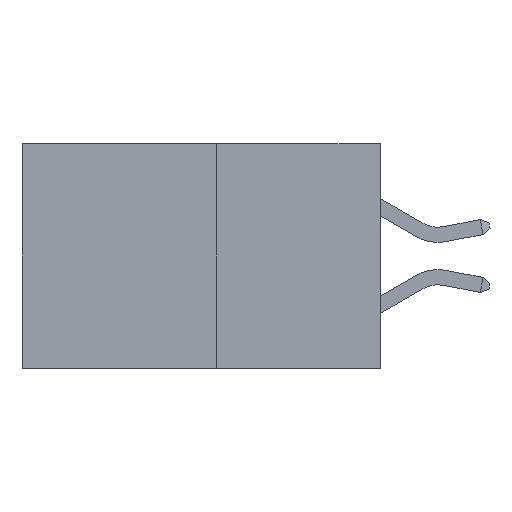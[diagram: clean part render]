
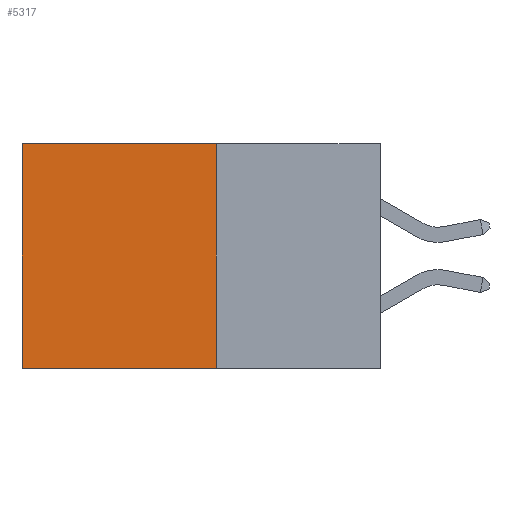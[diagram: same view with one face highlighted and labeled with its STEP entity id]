
A CAD part, left-side view. The second image highlights one B-rep face of the part: STEP entity #5317.
In plain terms, the highlighted planar face has unit normal (-1, 0, 0).
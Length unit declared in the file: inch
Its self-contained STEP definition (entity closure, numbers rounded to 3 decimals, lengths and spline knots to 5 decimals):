
#387 = DIRECTION ( 'NONE',  ( 0., 1., 0. ) ) ;
#841 = VECTOR ( 'NONE', #8076, 39.37008 ) ;
#886 = ORIENTED_EDGE ( 'NONE', *, *, #4565, .F. ) ;
#988 = AXIS2_PLACEMENT_3D ( 'NONE', #6729, #3667, #8965 ) ;
#1126 = VERTEX_POINT ( 'NONE', #8016 ) ;
#1153 = ORIENTED_EDGE ( 'NONE', *, *, #5943, .F. ) ;
#1343 = CARTESIAN_POINT ( 'NONE',  ( 0.277, 0.27, -0.37 ) ) ;
#1361 = ORIENTED_EDGE ( 'NONE', *, *, #4518, .T. ) ;
#2018 = CARTESIAN_POINT ( 'NONE',  ( 0.277, 0.27, -0.37 ) ) ;
#2144 = DIRECTION ( 'NONE',  ( 0., 0., -1. ) ) ;
#2391 = ORIENTED_EDGE ( 'NONE', *, *, #8601, .T. ) ;
#2939 = CARTESIAN_POINT ( 'NONE',  ( 0.277, 0.27, 0. ) ) ;
#3139 = VECTOR ( 'NONE', #387, 39.37008 ) ;
#3479 = CARTESIAN_POINT ( 'NONE',  ( 0.277, 0.59, 0. ) ) ;
#3667 = DIRECTION ( 'NONE',  ( 1., 0., 0. ) ) ;
#3730 = VECTOR ( 'NONE', #9463, 39.37008 ) ;
#3890 = VERTEX_POINT ( 'NONE', #3479 ) ;
#4222 = CARTESIAN_POINT ( 'NONE',  ( 0.277, 0.27, 0. ) ) ;
#4518 = EDGE_CURVE ( 'NONE', #4718, #3890, #5203, .T. ) ;
#4565 = EDGE_CURVE ( 'NONE', #9541, #1126, #6951, .T. ) ;
#4718 = VERTEX_POINT ( 'NONE', #2939 ) ;
#4746 = CARTESIAN_POINT ( 'NONE',  ( 0.277, 0.27, -0.37 ) ) ;
#5203 = LINE ( 'NONE', #4222, #3139 ) ;
#5317 = ADVANCED_FACE ( 'NONE', ( #6820 ), #8253, .F. ) ;
#5498 = LINE ( 'NONE', #1343, #9190 ) ;
#5943 = EDGE_CURVE ( 'NONE', #4718, #9541, #5498, .T. ) ;
#6531 = CARTESIAN_POINT ( 'NONE',  ( 0.277, 0.59, -0.37 ) ) ;
#6729 = CARTESIAN_POINT ( 'NONE',  ( 0.277, 0.27, -0.37 ) ) ;
#6820 = FACE_OUTER_BOUND ( 'NONE', #9131, .T. ) ;
#6951 = LINE ( 'NONE', #2018, #841 ) ;
#7812 = LINE ( 'NONE', #6531, #3730 ) ;
#8016 = CARTESIAN_POINT ( 'NONE',  ( 0.277, 0.59, -0.37 ) ) ;
#8076 = DIRECTION ( 'NONE',  ( 0., 1., 0. ) ) ;
#8253 = PLANE ( 'NONE',  #988 ) ;
#8601 = EDGE_CURVE ( 'NONE', #3890, #1126, #7812, .T. ) ;
#8965 = DIRECTION ( 'NONE',  ( 0., 0., -1. ) ) ;
#9131 = EDGE_LOOP ( 'NONE', ( #2391, #886, #1153, #1361 ) ) ;
#9190 = VECTOR ( 'NONE', #2144, 39.37008 ) ;
#9463 = DIRECTION ( 'NONE',  ( 0., 0., -1. ) ) ;
#9541 = VERTEX_POINT ( 'NONE', #4746 ) ;
